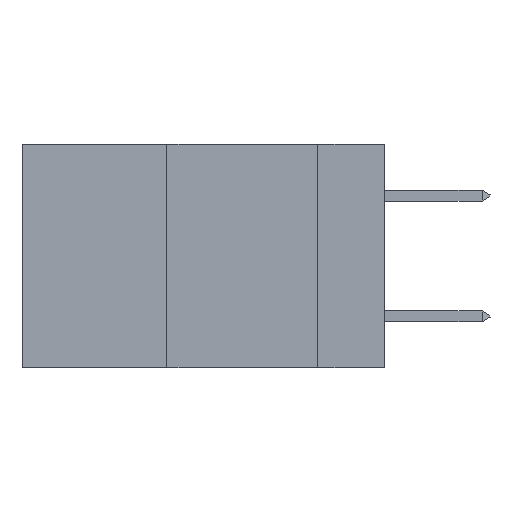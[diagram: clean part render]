
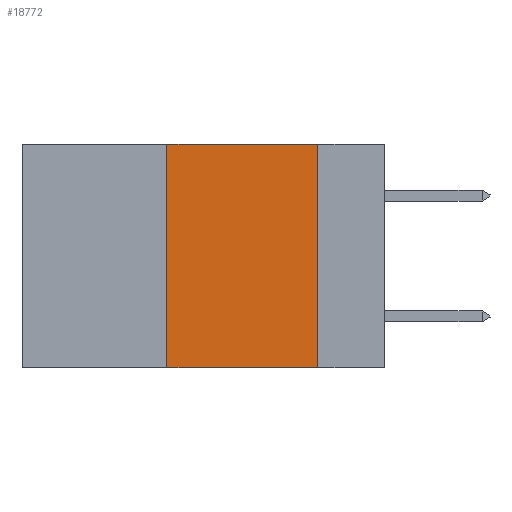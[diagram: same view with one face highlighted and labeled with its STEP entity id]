
A CAD part, left-side view. The second image highlights one B-rep face of the part: STEP entity #18772.
In plain terms, the highlighted planar face has unit normal (-1, 0, 0).
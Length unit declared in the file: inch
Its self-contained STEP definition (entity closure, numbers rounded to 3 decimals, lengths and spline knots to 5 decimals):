
#1373 = EDGE_LOOP ( 'NONE', ( #3603, #31105, #32119, #9285 ) ) ;
#2014 = CARTESIAN_POINT ( 'NONE',  ( 0., 0.11, 0. ) ) ;
#3541 = DIRECTION ( 'NONE',  ( 0., -1., 0. ) ) ;
#3603 = ORIENTED_EDGE ( 'NONE', *, *, #29158, .F. ) ;
#4548 = DIRECTION ( 'NONE',  ( 0., 0., -1. ) ) ;
#5000 = DIRECTION ( 'NONE',  ( 0., 0., -1. ) ) ;
#6984 = VECTOR ( 'NONE', #15377, 39.37008 ) ;
#7377 = VECTOR ( 'NONE', #25225, 39.37008 ) ;
#8831 = CARTESIAN_POINT ( 'NONE',  ( 0., 0.6, 0. ) ) ;
#9285 = ORIENTED_EDGE ( 'NONE', *, *, #14278, .T. ) ;
#10739 = CARTESIAN_POINT ( 'NONE',  ( 0., 0.36, 0. ) ) ;
#13108 = CARTESIAN_POINT ( 'NONE',  ( 0., 0.11, -0.37 ) ) ;
#13617 = VERTEX_POINT ( 'NONE', #10739 ) ;
#13992 = EDGE_CURVE ( 'NONE', #13617, #32677, #25286, .T. ) ;
#14114 = VECTOR ( 'NONE', #5000, 39.37008 ) ;
#14278 = EDGE_CURVE ( 'NONE', #25611, #34532, #31571, .T. ) ;
#14562 = CARTESIAN_POINT ( 'NONE',  ( 0., 0.36, -0.37 ) ) ;
#15377 = DIRECTION ( 'NONE',  ( 0., 0., 1. ) ) ;
#16560 = CARTESIAN_POINT ( 'NONE',  ( 0., 0.6, -0.37 ) ) ;
#17083 = FACE_OUTER_BOUND ( 'NONE', #1373, .T. ) ;
#17555 = PLANE ( 'NONE',  #24214 ) ;
#17679 = DIRECTION ( 'NONE',  ( 1., 0., 0. ) ) ;
#18772 = ADVANCED_FACE ( 'NONE', ( #17083 ), #17555, .F. ) ;
#21073 = CARTESIAN_POINT ( 'NONE',  ( 0., 0.6, 0. ) ) ;
#23545 = LINE ( 'NONE', #35626, #6984 ) ;
#24214 = AXIS2_PLACEMENT_3D ( 'NONE', #8831, #17679, #4548 ) ;
#25225 = DIRECTION ( 'NONE',  ( 0., -1., 0. ) ) ;
#25286 = LINE ( 'NONE', #21073, #32053 ) ;
#25611 = VERTEX_POINT ( 'NONE', #14562 ) ;
#27539 = CARTESIAN_POINT ( 'NONE',  ( 0., 0.11, 0. ) ) ;
#29158 = EDGE_CURVE ( 'NONE', #32677, #34532, #37191, .T. ) ;
#31105 = ORIENTED_EDGE ( 'NONE', *, *, #13992, .F. ) ;
#31571 = LINE ( 'NONE', #16560, #7377 ) ;
#31999 = EDGE_CURVE ( 'NONE', #25611, #13617, #23545, .T. ) ;
#32053 = VECTOR ( 'NONE', #3541, 39.37008 ) ;
#32119 = ORIENTED_EDGE ( 'NONE', *, *, #31999, .F. ) ;
#32677 = VERTEX_POINT ( 'NONE', #27539 ) ;
#34532 = VERTEX_POINT ( 'NONE', #13108 ) ;
#35626 = CARTESIAN_POINT ( 'NONE',  ( 0., 0.36, 0. ) ) ;
#37191 = LINE ( 'NONE', #2014, #14114 ) ;
